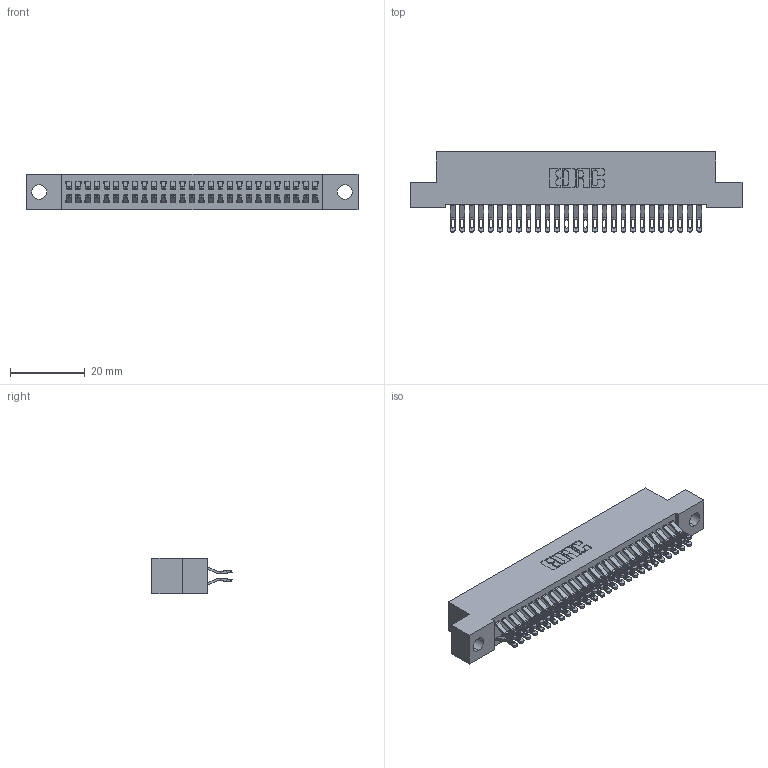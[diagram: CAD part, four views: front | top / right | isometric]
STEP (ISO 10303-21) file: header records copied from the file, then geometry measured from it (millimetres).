
FILE_DESCRIPTION (( 'STEP AP203' ), '1' );
FILE_NAME ('392-054-555-204.STEP', '2019-10-08T14:02:16', ( '' ), ( '' ), 'SwSTEP 2.0', 'SolidWorks 2016', '' );
FILE_SCHEMA (( 'CONFIG_CONTROL_DESIGN' ));
Length unit declared in the file: inch
Products named in the file (3): 392-054-555-204; 342 Part_.156 TH; 345-292-001_555 Tail
Assembly tree (55 placements, depth 2):
  392-054-555-204
    342 Part_.156 TH
    345-292-001_555 Tail  x54
Bounding box: 88.9 x 21.47 x 9.4 mm (x, y, z)
Volume: 7979.7 mm3; surface area: 12966 mm2
Topology: 55 solids, 55 shells, 3242 faces, 10181 edges, 6786 vertices
Faces by surface type: plane 1902, cylinder 1340
Entity records: 19507 total; most frequent: CARTESIAN_POINT 3284, ORIENTED_EDGE 3190, DIRECTION 2803, EDGE_CURVE 1595, VECTOR 1447, LINE 1447, VERTEX_POINT 1062, AXIS2_PLACEMENT_3D 678
